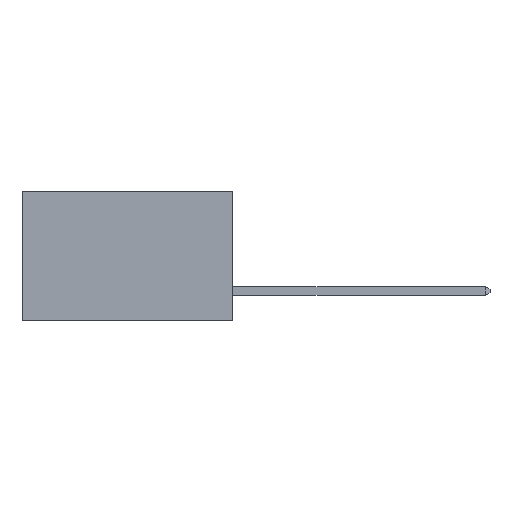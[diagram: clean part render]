
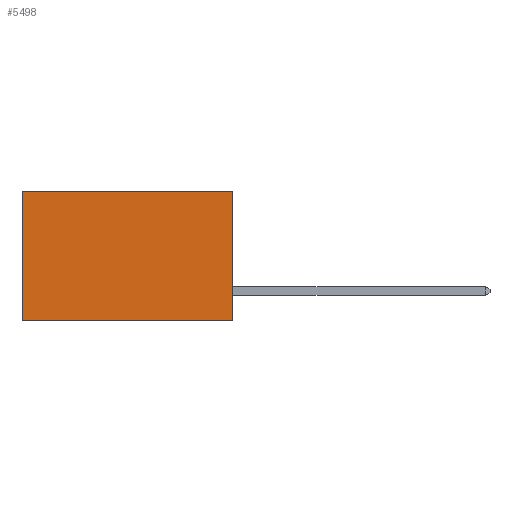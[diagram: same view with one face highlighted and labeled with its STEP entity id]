
A CAD part, left-side view. The second image highlights one B-rep face of the part: STEP entity #5498.
In plain terms, the highlighted planar face has unit normal (-1, 0, 0).
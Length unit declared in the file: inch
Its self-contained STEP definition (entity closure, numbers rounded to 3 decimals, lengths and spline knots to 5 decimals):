
#237 = VERTEX_POINT ( 'NONE', #1783 ) ;
#447 = ORIENTED_EDGE ( 'NONE', *, *, #6408, .T. ) ;
#609 = DIRECTION ( 'NONE',  ( 0., 0., -1. ) ) ;
#975 = DIRECTION ( 'NONE',  ( 1., 0., 0. ) ) ;
#1238 = LINE ( 'NONE', #8308, #5236 ) ;
#1671 = CARTESIAN_POINT ( 'NONE',  ( 0.2875, 0.6, 0. ) ) ;
#1783 = CARTESIAN_POINT ( 'NONE',  ( 0.2875, 0., -0.37 ) ) ;
#1891 = DIRECTION ( 'NONE',  ( 0., 0., -1. ) ) ;
#1919 = DIRECTION ( 'NONE',  ( 0., 1., 0. ) ) ;
#2155 = ORIENTED_EDGE ( 'NONE', *, *, #3266, .F. ) ;
#2401 = PLANE ( 'NONE',  #5334 ) ;
#2586 = EDGE_LOOP ( 'NONE', ( #10483, #8877, #2155, #447 ) ) ;
#2918 = CARTESIAN_POINT ( 'NONE',  ( 0.2875, 0.6, -0.37 ) ) ;
#3266 = EDGE_CURVE ( 'NONE', #7980, #237, #1238, .T. ) ;
#3836 = EDGE_CURVE ( 'NONE', #10027, #4146, #10588, .T. ) ;
#4146 = VERTEX_POINT ( 'NONE', #2918 ) ;
#4712 = CARTESIAN_POINT ( 'NONE',  ( 0.2875, 0., 0. ) ) ;
#5236 = VECTOR ( 'NONE', #609, 39.37008 ) ;
#5334 = AXIS2_PLACEMENT_3D ( 'NONE', #9072, #975, #1891 ) ;
#5498 = ADVANCED_FACE ( 'NONE', ( #9148 ), #2401, .F. ) ;
#5965 = VECTOR ( 'NONE', #1919, 39.37008 ) ;
#6389 = VECTOR ( 'NONE', #10907, 39.37008 ) ;
#6405 = LINE ( 'NONE', #10115, #8291 ) ;
#6408 = EDGE_CURVE ( 'NONE', #7980, #10027, #8120, .T. ) ;
#7980 = VERTEX_POINT ( 'NONE', #9250 ) ;
#8120 = LINE ( 'NONE', #4712, #5965 ) ;
#8291 = VECTOR ( 'NONE', #10887, 39.37008 ) ;
#8308 = CARTESIAN_POINT ( 'NONE',  ( 0.2875, 0., 0. ) ) ;
#8877 = ORIENTED_EDGE ( 'NONE', *, *, #9944, .F. ) ;
#9072 = CARTESIAN_POINT ( 'NONE',  ( 0.2875, 0., 0. ) ) ;
#9148 = FACE_OUTER_BOUND ( 'NONE', #2586, .T. ) ;
#9250 = CARTESIAN_POINT ( 'NONE',  ( 0.2875, 0., 0. ) ) ;
#9944 = EDGE_CURVE ( 'NONE', #237, #4146, #6405, .T. ) ;
#10027 = VERTEX_POINT ( 'NONE', #10213 ) ;
#10115 = CARTESIAN_POINT ( 'NONE',  ( 0.2875, 0., -0.37 ) ) ;
#10213 = CARTESIAN_POINT ( 'NONE',  ( 0.2875, 0.6, 0. ) ) ;
#10483 = ORIENTED_EDGE ( 'NONE', *, *, #3836, .T. ) ;
#10588 = LINE ( 'NONE', #1671, #6389 ) ;
#10887 = DIRECTION ( 'NONE',  ( 0., 1., 0. ) ) ;
#10907 = DIRECTION ( 'NONE',  ( 0., 0., -1. ) ) ;
